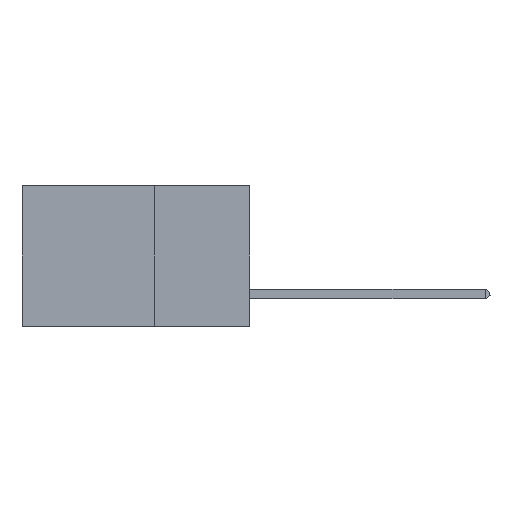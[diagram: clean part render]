
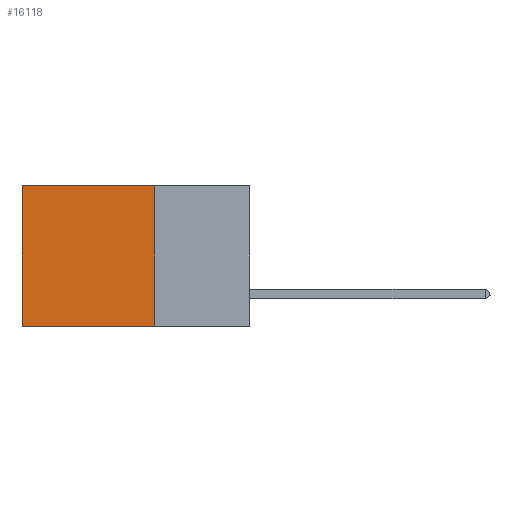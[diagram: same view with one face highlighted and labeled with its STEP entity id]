
A CAD part, left-side view. The second image highlights one B-rep face of the part: STEP entity #16118.
In plain terms, the highlighted planar face has unit normal (-1, 0, 0).
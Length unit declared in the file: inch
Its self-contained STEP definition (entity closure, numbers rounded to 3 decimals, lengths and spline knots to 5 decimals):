
#229 = CARTESIAN_POINT ( 'NONE',  ( 0.2875, 0.25, 0. ) ) ;
#646 = EDGE_CURVE ( 'NONE', #13473, #12959, #10153, .T. ) ;
#1468 = DIRECTION ( 'NONE',  ( 0., 0., -1. ) ) ;
#2366 = DIRECTION ( 'NONE',  ( 0., 1., 0. ) ) ;
#2489 = EDGE_CURVE ( 'NONE', #5984, #12959, #3742, .T. ) ;
#2613 = CARTESIAN_POINT ( 'NONE',  ( 0.2875, 0.25, -0.37 ) ) ;
#3089 = CARTESIAN_POINT ( 'NONE',  ( 0.2875, 0.6, 0. ) ) ;
#3742 = LINE ( 'NONE', #3089, #15919 ) ;
#4048 = VECTOR ( 'NONE', #2366, 39.37008 ) ;
#4322 = DIRECTION ( 'NONE',  ( 0., 1., 0. ) ) ;
#4955 = ORIENTED_EDGE ( 'NONE', *, *, #13684, .T. ) ;
#5283 = ORIENTED_EDGE ( 'NONE', *, *, #12388, .F. ) ;
#5414 = CARTESIAN_POINT ( 'NONE',  ( 0.2875, 0.6, -0.37 ) ) ;
#5737 = CARTESIAN_POINT ( 'NONE',  ( 0.2875, 0.25, 0. ) ) ;
#5984 = VERTEX_POINT ( 'NONE', #6625 ) ;
#6202 = LINE ( 'NONE', #5737, #14642 ) ;
#6625 = CARTESIAN_POINT ( 'NONE',  ( 0.2875, 0.6, 0. ) ) ;
#6977 = CARTESIAN_POINT ( 'NONE',  ( 0.2875, 0.25, -0.37 ) ) ;
#8048 = CARTESIAN_POINT ( 'NONE',  ( 0.2875, 0.25, 0. ) ) ;
#8266 = EDGE_LOOP ( 'NONE', ( #8278, #8710, #5283, #4955 ) ) ;
#8278 = ORIENTED_EDGE ( 'NONE', *, *, #2489, .T. ) ;
#8710 = ORIENTED_EDGE ( 'NONE', *, *, #646, .F. ) ;
#8938 = FACE_OUTER_BOUND ( 'NONE', #8266, .T. ) ;
#9372 = VERTEX_POINT ( 'NONE', #8048 ) ;
#10153 = LINE ( 'NONE', #2613, #4048 ) ;
#10689 = CARTESIAN_POINT ( 'NONE',  ( 0.2875, 0.25, 0. ) ) ;
#11423 = AXIS2_PLACEMENT_3D ( 'NONE', #229, #14188, #14122 ) ;
#12106 = DIRECTION ( 'NONE',  ( 0., 0., -1. ) ) ;
#12388 = EDGE_CURVE ( 'NONE', #9372, #13473, #16819, .T. ) ;
#12822 = PLANE ( 'NONE',  #11423 ) ;
#12959 = VERTEX_POINT ( 'NONE', #5414 ) ;
#13473 = VERTEX_POINT ( 'NONE', #6977 ) ;
#13684 = EDGE_CURVE ( 'NONE', #9372, #5984, #6202, .T. ) ;
#14021 = VECTOR ( 'NONE', #12106, 39.37008 ) ;
#14122 = DIRECTION ( 'NONE',  ( 0., 0., -1. ) ) ;
#14188 = DIRECTION ( 'NONE',  ( 1., 0., 0. ) ) ;
#14642 = VECTOR ( 'NONE', #4322, 39.37008 ) ;
#15919 = VECTOR ( 'NONE', #1468, 39.37008 ) ;
#16118 = ADVANCED_FACE ( 'NONE', ( #8938 ), #12822, .F. ) ;
#16819 = LINE ( 'NONE', #10689, #14021 ) ;
